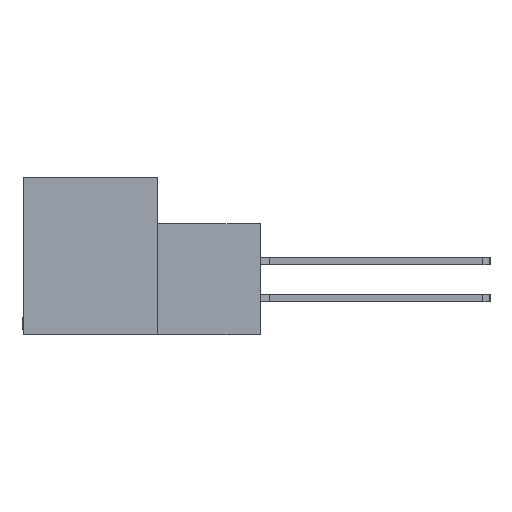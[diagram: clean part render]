
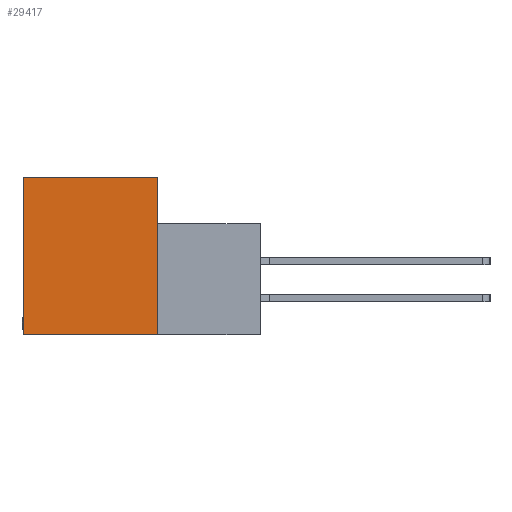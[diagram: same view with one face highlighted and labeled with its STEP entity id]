
A CAD part, left-side view. The second image highlights one B-rep face of the part: STEP entity #29417.
In plain terms, the highlighted planar face has unit normal (-1, 0, 0).
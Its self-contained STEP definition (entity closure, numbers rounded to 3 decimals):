
#1379 = CARTESIAN_POINT ( 'NONE',  ( 0., 0., 0. ) ) ;
#2604 = LINE ( 'NONE', #29921, #10888 ) ;
#2714 = CARTESIAN_POINT ( 'NONE',  ( 0., 11.506, -13.487 ) ) ;
#2746 = LINE ( 'NONE', #41638, #3920 ) ;
#3920 = VECTOR ( 'NONE', #9381, 1000. ) ;
#5042 = VECTOR ( 'NONE', #12366, 1000. ) ;
#7995 = ORIENTED_EDGE ( 'NONE', *, *, #42809, .F. ) ;
#8481 = DIRECTION ( 'NONE',  ( 0., 0., -1. ) ) ;
#9381 = DIRECTION ( 'NONE',  ( 0., 0., 1. ) ) ;
#10835 = CARTESIAN_POINT ( 'NONE',  ( 0., -8.814, -13.487 ) ) ;
#10888 = VECTOR ( 'NONE', #29452, 1000. ) ;
#10983 = DIRECTION ( 'NONE',  ( 0., 1., 0. ) ) ;
#11982 = VERTEX_POINT ( 'NONE', #2714 ) ;
#12366 = DIRECTION ( 'NONE',  ( 0., 0., -1. ) ) ;
#12484 = AXIS2_PLACEMENT_3D ( 'NONE', #1379, #39616, #8481 ) ;
#17560 = VERTEX_POINT ( 'NONE', #32091 ) ;
#17576 = EDGE_CURVE ( 'NONE', #17560, #11982, #23148, .T. ) ;
#17626 = VECTOR ( 'NONE', #10983, 1000. ) ;
#22103 = CARTESIAN_POINT ( 'NONE',  ( 0., 11.506, 0. ) ) ;
#22481 = PLANE ( 'NONE',  #12484 ) ;
#23148 = LINE ( 'NONE', #10835, #17626 ) ;
#24616 = EDGE_CURVE ( 'NONE', #35740, #44530, #2604, .T. ) ;
#27508 = FACE_OUTER_BOUND ( 'NONE', #27817, .T. ) ;
#27817 = EDGE_LOOP ( 'NONE', ( #29427, #29596, #44681, #7995 ) ) ;
#29417 = ADVANCED_FACE ( 'NONE', ( #27508 ), #22481, .F. ) ;
#29427 = ORIENTED_EDGE ( 'NONE', *, *, #17576, .F. ) ;
#29452 = DIRECTION ( 'NONE',  ( 0., -1., 0. ) ) ;
#29596 = ORIENTED_EDGE ( 'NONE', *, *, #45666, .F. ) ;
#29921 = CARTESIAN_POINT ( 'NONE',  ( 0., 11.506, 0. ) ) ;
#30430 = LINE ( 'NONE', #32700, #5042 ) ;
#32091 = CARTESIAN_POINT ( 'NONE',  ( 0., 0., -13.487 ) ) ;
#32700 = CARTESIAN_POINT ( 'NONE',  ( 0., 0., 0. ) ) ;
#33250 = CARTESIAN_POINT ( 'NONE',  ( 0., 0., 0. ) ) ;
#35740 = VERTEX_POINT ( 'NONE', #22103 ) ;
#39616 = DIRECTION ( 'NONE',  ( 1., 0., 0. ) ) ;
#41638 = CARTESIAN_POINT ( 'NONE',  ( 0., 11.506, -13.487 ) ) ;
#42809 = EDGE_CURVE ( 'NONE', #11982, #35740, #2746, .T. ) ;
#44530 = VERTEX_POINT ( 'NONE', #33250 ) ;
#44681 = ORIENTED_EDGE ( 'NONE', *, *, #24616, .F. ) ;
#45666 = EDGE_CURVE ( 'NONE', #44530, #17560, #30430, .T. ) ;
